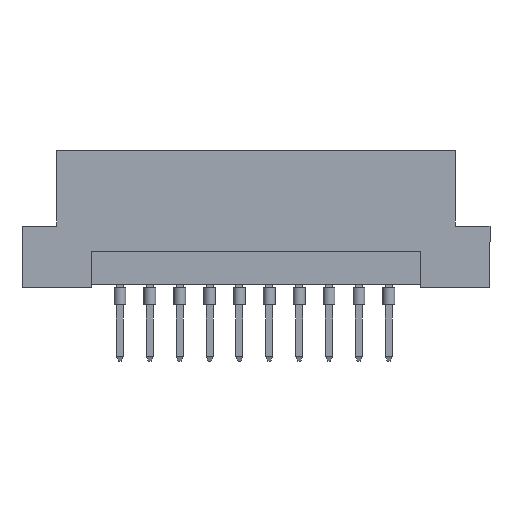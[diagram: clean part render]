
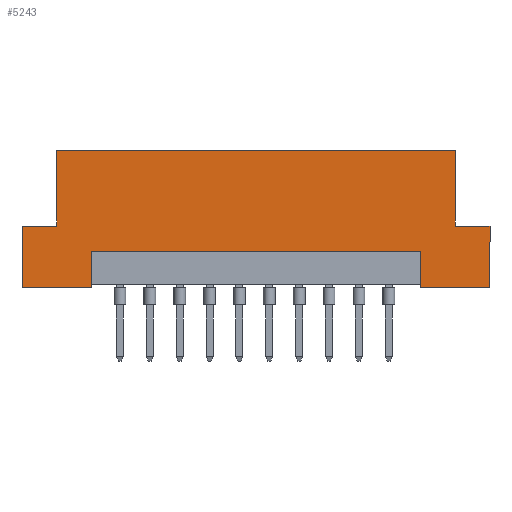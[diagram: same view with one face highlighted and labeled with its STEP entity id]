
A CAD part, front view. The second image highlights one B-rep face of the part: STEP entity #5243.
In plain terms, the highlighted planar face has unit normal (0, -1, 0).
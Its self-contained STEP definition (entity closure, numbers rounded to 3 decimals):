
#13 = EDGE_CURVE ( 'NONE', #2945, #3578, #4724, .T. ) ;
#92 = VERTEX_POINT ( 'NONE', #1342 ) ;
#130 = ORIENTED_EDGE ( 'NONE', *, *, #1017, .F. ) ;
#158 = EDGE_CURVE ( 'NONE', #4930, #2679, #1908, .T. ) ;
#210 = VERTEX_POINT ( 'NONE', #1589 ) ;
#219 = ORIENTED_EDGE ( 'NONE', *, *, #839, .T. ) ;
#323 = VECTOR ( 'NONE', #3355, 1000. ) ;
#383 = LINE ( 'NONE', #640, #4937 ) ;
#483 = DIRECTION ( 'NONE',  ( 0., 1., 0. ) ) ;
#547 = CARTESIAN_POINT ( 'NONE',  ( -14., -4.3, 0. ) ) ;
#612 = CARTESIAN_POINT ( 'NONE',  ( 19.9, -4.3, 11.6 ) ) ;
#640 = CARTESIAN_POINT ( 'NONE',  ( 19.9, -4.3, 5.2 ) ) ;
#839 = EDGE_CURVE ( 'NONE', #5166, #2679, #4187, .T. ) ;
#854 = CARTESIAN_POINT ( 'NONE',  ( -19.9, -4.3, 5.2 ) ) ;
#925 = VECTOR ( 'NONE', #1368, 1000. ) ;
#1017 = EDGE_CURVE ( 'NONE', #4326, #210, #4770, .T. ) ;
#1034 = CARTESIAN_POINT ( 'NONE',  ( 19.9, -4.3, 0. ) ) ;
#1055 = EDGE_CURVE ( 'NONE', #2945, #3530, #4946, .T. ) ;
#1168 = VECTOR ( 'NONE', #2829, 1000. ) ;
#1342 = CARTESIAN_POINT ( 'NONE',  ( -14., -4.3, 3. ) ) ;
#1347 = DIRECTION ( 'NONE',  ( 0., 0., -1. ) ) ;
#1368 = DIRECTION ( 'NONE',  ( 0., 0., -1. ) ) ;
#1435 = DIRECTION ( 'NONE',  ( 1., 0., 0. ) ) ;
#1447 = CARTESIAN_POINT ( 'NONE',  ( 19.9, -4.3, 11.6 ) ) ;
#1496 = VECTOR ( 'NONE', #5400, 1000. ) ;
#1589 = CARTESIAN_POINT ( 'NONE',  ( -16.94, -4.3, 5.2 ) ) ;
#1591 = AXIS2_PLACEMENT_3D ( 'NONE', #3152, #483, #4924 ) ;
#1600 = CARTESIAN_POINT ( 'NONE',  ( 19.9, -4.3, 0. ) ) ;
#1602 = ORIENTED_EDGE ( 'NONE', *, *, #5010, .F. ) ;
#1819 = DIRECTION ( 'NONE',  ( 1., 0., 0. ) ) ;
#1823 = ORIENTED_EDGE ( 'NONE', *, *, #2592, .F. ) ;
#1834 = VECTOR ( 'NONE', #1819, 1000. ) ;
#1844 = ORIENTED_EDGE ( 'NONE', *, *, #13, .T. ) ;
#1863 = CARTESIAN_POINT ( 'NONE',  ( 16.94, -4.3, 11.6 ) ) ;
#1884 = FACE_OUTER_BOUND ( 'NONE', #4859, .T. ) ;
#1908 = LINE ( 'NONE', #1447, #1168 ) ;
#1999 = CARTESIAN_POINT ( 'NONE',  ( -19.9, -4.3, 5.2 ) ) ;
#2235 = VERTEX_POINT ( 'NONE', #3129 ) ;
#2264 = ORIENTED_EDGE ( 'NONE', *, *, #5566, .T. ) ;
#2347 = LINE ( 'NONE', #4096, #1834 ) ;
#2419 = CARTESIAN_POINT ( 'NONE',  ( -16.94, -4.3, 11.6 ) ) ;
#2451 = VERTEX_POINT ( 'NONE', #4791 ) ;
#2592 = EDGE_CURVE ( 'NONE', #2235, #3578, #4872, .T. ) ;
#2602 = DIRECTION ( 'NONE',  ( 1., 0., 0. ) ) ;
#2612 = VECTOR ( 'NONE', #5265, 1000. ) ;
#2679 = VERTEX_POINT ( 'NONE', #1863 ) ;
#2773 = ORIENTED_EDGE ( 'NONE', *, *, #4622, .F. ) ;
#2774 = ORIENTED_EDGE ( 'NONE', *, *, #158, .F. ) ;
#2829 = DIRECTION ( 'NONE',  ( 1., 0., 0. ) ) ;
#2945 = VERTEX_POINT ( 'NONE', #3477 ) ;
#3064 = VECTOR ( 'NONE', #5470, 1000. ) ;
#3094 = CARTESIAN_POINT ( 'NONE',  ( -19.9, -4.3, 11.6 ) ) ;
#3129 = CARTESIAN_POINT ( 'NONE',  ( 19.9, -4.3, 5.2 ) ) ;
#3152 = CARTESIAN_POINT ( 'NONE',  ( 19.9, -4.3, 11.6 ) ) ;
#3321 = CARTESIAN_POINT ( 'NONE',  ( -16.94, -4.3, 5.2 ) ) ;
#3355 = DIRECTION ( 'NONE',  ( 1., 0., 0. ) ) ;
#3427 = VECTOR ( 'NONE', #1347, 1000. ) ;
#3433 = VECTOR ( 'NONE', #2602, 1000. ) ;
#3477 = CARTESIAN_POINT ( 'NONE',  ( 14., -4.3, 0. ) ) ;
#3530 = VERTEX_POINT ( 'NONE', #4807 ) ;
#3543 = ORIENTED_EDGE ( 'NONE', *, *, #5527, .T. ) ;
#3578 = VERTEX_POINT ( 'NONE', #1034 ) ;
#3598 = LINE ( 'NONE', #3094, #925 ) ;
#3660 = VECTOR ( 'NONE', #5098, 1000. ) ;
#3714 = EDGE_CURVE ( 'NONE', #210, #4930, #5357, .T. ) ;
#3733 = ORIENTED_EDGE ( 'NONE', *, *, #1055, .F. ) ;
#3841 = VECTOR ( 'NONE', #3925, 1000. ) ;
#3925 = DIRECTION ( 'NONE',  ( 1., 0., 0. ) ) ;
#4068 = CARTESIAN_POINT ( 'NONE',  ( 16.94, -4.3, 5.2 ) ) ;
#4096 = CARTESIAN_POINT ( 'NONE',  ( -14., -4.3, 3. ) ) ;
#4107 = ORIENTED_EDGE ( 'NONE', *, *, #3714, .F. ) ;
#4187 = LINE ( 'NONE', #5013, #3064 ) ;
#4262 = LINE ( 'NONE', #4319, #3841 ) ;
#4319 = CARTESIAN_POINT ( 'NONE',  ( 19.9, -4.3, 0. ) ) ;
#4326 = VERTEX_POINT ( 'NONE', #1999 ) ;
#4491 = PLANE ( 'NONE',  #1591 ) ;
#4622 = EDGE_CURVE ( 'NONE', #5166, #2235, #383, .T. ) ;
#4658 = VERTEX_POINT ( 'NONE', #547 ) ;
#4724 = LINE ( 'NONE', #1600, #323 ) ;
#4730 = LINE ( 'NONE', #5275, #3427 ) ;
#4770 = LINE ( 'NONE', #854, #3433 ) ;
#4791 = CARTESIAN_POINT ( 'NONE',  ( -19.9, -4.3, 0. ) ) ;
#4807 = CARTESIAN_POINT ( 'NONE',  ( 14., -4.3, 3. ) ) ;
#4859 = EDGE_LOOP ( 'NONE', ( #2264, #3733, #1844, #1823, #2773, #219, #2774, #4107, #130, #5508, #3543, #1602 ) ) ;
#4872 = LINE ( 'NONE', #612, #1496 ) ;
#4924 = DIRECTION ( 'NONE',  ( -1., 0., 0. ) ) ;
#4930 = VERTEX_POINT ( 'NONE', #2419 ) ;
#4937 = VECTOR ( 'NONE', #1435, 1000. ) ;
#4946 = LINE ( 'NONE', #5320, #2612 ) ;
#5010 = EDGE_CURVE ( 'NONE', #92, #4658, #4730, .T. ) ;
#5013 = CARTESIAN_POINT ( 'NONE',  ( 16.94, -4.3, 5.2 ) ) ;
#5098 = DIRECTION ( 'NONE',  ( 0., 0., 1. ) ) ;
#5166 = VERTEX_POINT ( 'NONE', #4068 ) ;
#5243 = ADVANCED_FACE ( 'NONE', ( #1884 ), #4491, .F. ) ;
#5265 = DIRECTION ( 'NONE',  ( 0., 0., 1. ) ) ;
#5275 = CARTESIAN_POINT ( 'NONE',  ( -14., -4.3, 0.2 ) ) ;
#5320 = CARTESIAN_POINT ( 'NONE',  ( 14., -4.3, 0.2 ) ) ;
#5357 = LINE ( 'NONE', #3321, #3660 ) ;
#5400 = DIRECTION ( 'NONE',  ( 0., 0., -1. ) ) ;
#5470 = DIRECTION ( 'NONE',  ( 0., 0., 1. ) ) ;
#5508 = ORIENTED_EDGE ( 'NONE', *, *, #5664, .T. ) ;
#5527 = EDGE_CURVE ( 'NONE', #2451, #4658, #4262, .T. ) ;
#5566 = EDGE_CURVE ( 'NONE', #92, #3530, #2347, .T. ) ;
#5664 = EDGE_CURVE ( 'NONE', #4326, #2451, #3598, .T. ) ;
